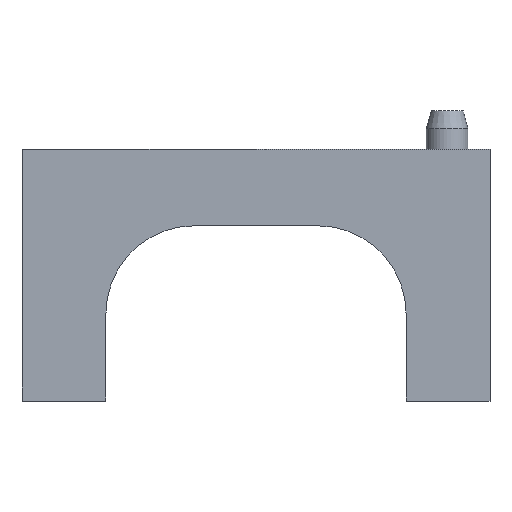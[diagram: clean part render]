
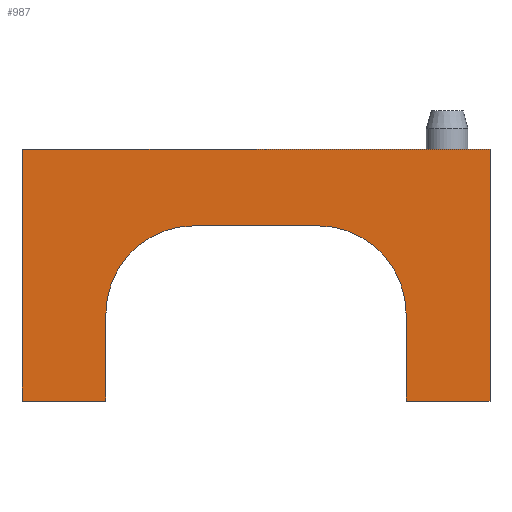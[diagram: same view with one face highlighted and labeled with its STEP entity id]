
A CAD part, front view. The second image highlights one B-rep face of the part: STEP entity #987.
In plain terms, the highlighted planar face has unit normal (0, -1, 0).
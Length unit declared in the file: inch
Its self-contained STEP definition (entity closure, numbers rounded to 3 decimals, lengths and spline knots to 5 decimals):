
#52 = DIRECTION ( 'NONE',  ( -1., 0., 0. ) ) ;
#81 = ORIENTED_EDGE ( 'NONE', *, *, #1077, .F. ) ;
#97 = VECTOR ( 'NONE', #720, 39.37008 ) ;
#128 = CIRCLE ( 'NONE', #233, 0.2 ) ;
#182 = PLANE ( 'NONE',  #476 ) ;
#233 = AXIS2_PLACEMENT_3D ( 'NONE', #1409, #1252, #1911 ) ;
#244 = ORIENTED_EDGE ( 'NONE', *, *, #1164, .F. ) ;
#258 = CARTESIAN_POINT ( 'NONE',  ( 0.34, -0.1425, -0.397 ) ) ;
#315 = EDGE_CURVE ( 'NONE', #1220, #1559, #1238, .T. ) ;
#320 = ORIENTED_EDGE ( 'NONE', *, *, #1422, .F. ) ;
#332 = ORIENTED_EDGE ( 'NONE', *, *, #335, .F. ) ;
#335 = EDGE_CURVE ( 'NONE', #1559, #1651, #2064, .T. ) ;
#356 = FACE_OUTER_BOUND ( 'NONE', #506, .T. ) ;
#375 = DIRECTION ( 'NONE',  ( 0., 0., 1. ) ) ;
#377 = CARTESIAN_POINT ( 'NONE',  ( -0.34, -0.1425, -0.2 ) ) ;
#395 = EDGE_CURVE ( 'NONE', #452, #1621, #1423, .T. ) ;
#398 = LINE ( 'NONE', #1047, #459 ) ;
#402 = EDGE_CURVE ( 'NONE', #1689, #452, #1370, .T. ) ;
#452 = VERTEX_POINT ( 'NONE', #1122 ) ;
#455 = AXIS2_PLACEMENT_3D ( 'NONE', #816, #479, #1145 ) ;
#459 = VECTOR ( 'NONE', #52, 39.37008 ) ;
#476 = AXIS2_PLACEMENT_3D ( 'NONE', #979, #1515, #375 ) ;
#479 = DIRECTION ( 'NONE',  ( 0., -1., 0. ) ) ;
#506 = EDGE_LOOP ( 'NONE', ( #332, #799, #320, #81, #244, #592, #1092, #1715, #961, #640 ) ) ;
#519 = VERTEX_POINT ( 'NONE', #377 ) ;
#560 = VECTOR ( 'NONE', #1654, 39.37008 ) ;
#592 = ORIENTED_EDGE ( 'NONE', *, *, #395, .F. ) ;
#625 = CARTESIAN_POINT ( 'NONE',  ( -0.34, -0.1425, -0.397 ) ) ;
#640 = ORIENTED_EDGE ( 'NONE', *, *, #1776, .F. ) ;
#688 = VECTOR ( 'NONE', #1748, 39.37008 ) ;
#720 = DIRECTION ( 'NONE',  ( 0., 0., -1. ) ) ;
#799 = ORIENTED_EDGE ( 'NONE', *, *, #315, .F. ) ;
#805 = LINE ( 'NONE', #1797, #560 ) ;
#816 = CARTESIAN_POINT ( 'NONE',  ( 0.14, -0.1425, -0.2 ) ) ;
#885 = DIRECTION ( 'NONE',  ( 1., 0., 0. ) ) ;
#891 = LINE ( 'NONE', #1071, #97 ) ;
#961 = ORIENTED_EDGE ( 'NONE', *, *, #1388, .F. ) ;
#979 = CARTESIAN_POINT ( 'NONE',  ( 0.14, -0.1425, -0.2 ) ) ;
#987 = ADVANCED_FACE ( 'NONE', ( #356 ), #182, .F. ) ;
#1037 = DIRECTION ( 'NONE',  ( -1., 0., 0. ) ) ;
#1047 = CARTESIAN_POINT ( 'NONE',  ( -0.34, -0.1425, -0.397 ) ) ;
#1071 = CARTESIAN_POINT ( 'NONE',  ( -0.34, -0.1425, -0.2 ) ) ;
#1077 = EDGE_CURVE ( 'NONE', #519, #1751, #891, .T. ) ;
#1088 = CARTESIAN_POINT ( 'NONE',  ( -0.53, -0.1425, 0.173 ) ) ;
#1092 = ORIENTED_EDGE ( 'NONE', *, *, #402, .F. ) ;
#1119 = CARTESIAN_POINT ( 'NONE',  ( 0.53, -0.1425, -0.397 ) ) ;
#1122 = CARTESIAN_POINT ( 'NONE',  ( 0.14, -0.1425, 0. ) ) ;
#1145 = DIRECTION ( 'NONE',  ( 0., 0., 1. ) ) ;
#1164 = EDGE_CURVE ( 'NONE', #1621, #519, #128, .T. ) ;
#1184 = CARTESIAN_POINT ( 'NONE',  ( 0.34, -0.1425, -0.2 ) ) ;
#1193 = CARTESIAN_POINT ( 'NONE',  ( -0.14, -0.1425, 0. ) ) ;
#1220 = VERTEX_POINT ( 'NONE', #1813 ) ;
#1238 = LINE ( 'NONE', #1896, #1516 ) ;
#1252 = DIRECTION ( 'NONE',  ( 0., -1., 0. ) ) ;
#1278 = VERTEX_POINT ( 'NONE', #258 ) ;
#1370 = CIRCLE ( 'NONE', #455, 0.2 ) ;
#1388 = EDGE_CURVE ( 'NONE', #1438, #1278, #1551, .T. ) ;
#1409 = CARTESIAN_POINT ( 'NONE',  ( -0.14, -0.1425, -0.2 ) ) ;
#1413 = LINE ( 'NONE', #1767, #688 ) ;
#1422 = EDGE_CURVE ( 'NONE', #1751, #1220, #398, .T. ) ;
#1423 = LINE ( 'NONE', #1941, #2022 ) ;
#1438 = VERTEX_POINT ( 'NONE', #1119 ) ;
#1515 = DIRECTION ( 'NONE',  ( 0., 1., 0. ) ) ;
#1516 = VECTOR ( 'NONE', #1872, 39.37008 ) ;
#1542 = CARTESIAN_POINT ( 'NONE',  ( 0.53, -0.1425, 0.173 ) ) ;
#1551 = LINE ( 'NONE', #1869, #2094 ) ;
#1559 = VERTEX_POINT ( 'NONE', #1951 ) ;
#1621 = VERTEX_POINT ( 'NONE', #1193 ) ;
#1651 = VERTEX_POINT ( 'NONE', #1542 ) ;
#1654 = DIRECTION ( 'NONE',  ( 0., 0., 1. ) ) ;
#1689 = VERTEX_POINT ( 'NONE', #1184 ) ;
#1715 = ORIENTED_EDGE ( 'NONE', *, *, #1839, .F. ) ;
#1748 = DIRECTION ( 'NONE',  ( 0., 0., -1. ) ) ;
#1751 = VERTEX_POINT ( 'NONE', #625 ) ;
#1767 = CARTESIAN_POINT ( 'NONE',  ( 0.53, -0.1425, -0.397 ) ) ;
#1776 = EDGE_CURVE ( 'NONE', #1651, #1438, #1413, .T. ) ;
#1797 = CARTESIAN_POINT ( 'NONE',  ( 0.34, -0.1425, -0.2 ) ) ;
#1813 = CARTESIAN_POINT ( 'NONE',  ( -0.53, -0.1425, -0.397 ) ) ;
#1819 = VECTOR ( 'NONE', #885, 39.37008 ) ;
#1839 = EDGE_CURVE ( 'NONE', #1278, #1689, #805, .T. ) ;
#1869 = CARTESIAN_POINT ( 'NONE',  ( 0.34, -0.1425, -0.397 ) ) ;
#1872 = DIRECTION ( 'NONE',  ( 0., 0., 1. ) ) ;
#1896 = CARTESIAN_POINT ( 'NONE',  ( -0.53, -0.1425, -0.397 ) ) ;
#1911 = DIRECTION ( 'NONE',  ( 0., 0., -1. ) ) ;
#1933 = DIRECTION ( 'NONE',  ( -1., 0., 0. ) ) ;
#1941 = CARTESIAN_POINT ( 'NONE',  ( 0.14, -0.1425, 0. ) ) ;
#1951 = CARTESIAN_POINT ( 'NONE',  ( -0.53, -0.1425, 0.173 ) ) ;
#2022 = VECTOR ( 'NONE', #1933, 39.37008 ) ;
#2064 = LINE ( 'NONE', #1088, #1819 ) ;
#2094 = VECTOR ( 'NONE', #1037, 39.37008 ) ;
